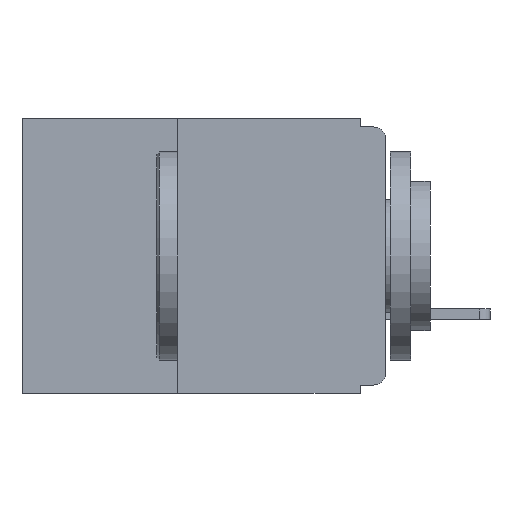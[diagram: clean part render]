
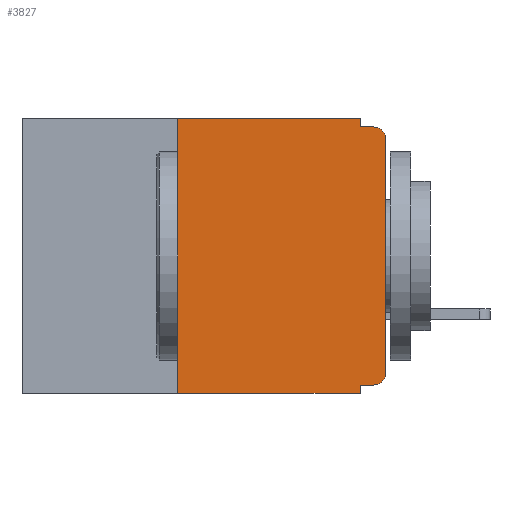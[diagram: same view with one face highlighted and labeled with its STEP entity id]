
A CAD part, left-side view. The second image highlights one B-rep face of the part: STEP entity #3827.
In plain terms, the highlighted planar face has unit normal (-1, 0, 0).
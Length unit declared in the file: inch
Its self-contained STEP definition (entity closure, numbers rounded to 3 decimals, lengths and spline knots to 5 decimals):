
#348 = AXIS2_PLACEMENT_3D ( 'NONE', #14447, #14427, #15139 ) ;
#410 = VECTOR ( 'NONE', #9246, 39.37008 ) ;
#411 = EDGE_CURVE ( 'NONE', #6225, #6337, #15366, .T. ) ;
#481 = ORIENTED_EDGE ( 'NONE', *, *, #848, .F. ) ;
#543 = EDGE_CURVE ( 'NONE', #963, #13553, #2872, .T. ) ;
#816 = CARTESIAN_POINT ( 'NONE',  ( 0., 0.437, 0. ) ) ;
#827 = LINE ( 'NONE', #11089, #410 ) ;
#848 = EDGE_CURVE ( 'NONE', #14130, #13197, #3654, .T. ) ;
#916 = VERTEX_POINT ( 'NONE', #8797 ) ;
#923 = EDGE_CURVE ( 'NONE', #6337, #13553, #6423, .T. ) ;
#963 = VERTEX_POINT ( 'NONE', #6775 ) ;
#1004 = EDGE_CURVE ( 'NONE', #14130, #6225, #8576, .T. ) ;
#1353 = CARTESIAN_POINT ( 'NONE',  ( 0., 0.031, 0. ) ) ;
#1358 = AXIS2_PLACEMENT_3D ( 'NONE', #3592, #9985, #3199 ) ;
#2254 = VECTOR ( 'NONE', #15752, 39.37008 ) ;
#2474 = VECTOR ( 'NONE', #9065, 39.37008 ) ;
#2872 = LINE ( 'NONE', #10908, #2474 ) ;
#2999 = ORIENTED_EDGE ( 'NONE', *, *, #923, .T. ) ;
#3199 = DIRECTION ( 'NONE',  ( 0., 0., -1. ) ) ;
#3592 = CARTESIAN_POINT ( 'NONE',  ( 0., 0.015, -0.025 ) ) ;
#3654 = LINE ( 'NONE', #4986, #13176 ) ;
#3827 = ADVANCED_FACE ( 'NONE', ( #10230 ), #13793, .F. ) ;
#4986 = CARTESIAN_POINT ( 'NONE',  ( 0., 0., -0.32 ) ) ;
#5029 = CARTESIAN_POINT ( 'NONE',  ( 0., 0., 0. ) ) ;
#5352 = ORIENTED_EDGE ( 'NONE', *, *, #5607, .F. ) ;
#5473 = LINE ( 'NONE', #12480, #11760 ) ;
#5557 = EDGE_CURVE ( 'NONE', #13282, #963, #5473, .T. ) ;
#5607 = EDGE_CURVE ( 'NONE', #916, #11730, #8041, .T. ) ;
#5628 = EDGE_CURVE ( 'NONE', #916, #6317, #827, .T. ) ;
#5681 = EDGE_CURVE ( 'NONE', #13197, #6317, #15749, .T. ) ;
#5975 = EDGE_LOOP ( 'NONE', ( #8987, #2999, #11660, #7120, #13309, #5352, #10160, #14050, #481, #10269 ) ) ;
#6225 = VERTEX_POINT ( 'NONE', #10763 ) ;
#6317 = VERTEX_POINT ( 'NONE', #9781 ) ;
#6337 = VERTEX_POINT ( 'NONE', #6688 ) ;
#6423 = CIRCLE ( 'NONE', #1358, 0.015 ) ;
#6459 = VECTOR ( 'NONE', #11538, 39.37008 ) ;
#6688 = CARTESIAN_POINT ( 'NONE',  ( 0., 0., -0.025 ) ) ;
#6775 = CARTESIAN_POINT ( 'NONE',  ( 0., 0.031, -0.01 ) ) ;
#7120 = ORIENTED_EDGE ( 'NONE', *, *, #5557, .F. ) ;
#7586 = DIRECTION ( 'NONE',  ( 0., 0., 1. ) ) ;
#7600 = CARTESIAN_POINT ( 'NONE',  ( 0., 0.031, -0.32 ) ) ;
#8041 = LINE ( 'NONE', #8678, #13791 ) ;
#8576 = CIRCLE ( 'NONE', #348, 0.015 ) ;
#8678 = CARTESIAN_POINT ( 'NONE',  ( 0., 0.25, -0.33 ) ) ;
#8797 = CARTESIAN_POINT ( 'NONE',  ( 0., 0.25, -0.33 ) ) ;
#8987 = ORIENTED_EDGE ( 'NONE', *, *, #411, .T. ) ;
#9065 = DIRECTION ( 'NONE',  ( 0., -1., 0. ) ) ;
#9246 = DIRECTION ( 'NONE',  ( 0., -1., 0. ) ) ;
#9781 = CARTESIAN_POINT ( 'NONE',  ( 0., 0.031, -0.33 ) ) ;
#9985 = DIRECTION ( 'NONE',  ( -1., 0., 0. ) ) ;
#10095 = CARTESIAN_POINT ( 'NONE',  ( 0., 0.015, -0.32 ) ) ;
#10146 = EDGE_CURVE ( 'NONE', #11730, #13282, #13825, .T. ) ;
#10160 = ORIENTED_EDGE ( 'NONE', *, *, #5628, .T. ) ;
#10230 = FACE_OUTER_BOUND ( 'NONE', #5975, .T. ) ;
#10269 = ORIENTED_EDGE ( 'NONE', *, *, #1004, .T. ) ;
#10763 = CARTESIAN_POINT ( 'NONE',  ( 0., 0., -0.305 ) ) ;
#10908 = CARTESIAN_POINT ( 'NONE',  ( 0., 0., -0.01 ) ) ;
#11089 = CARTESIAN_POINT ( 'NONE',  ( 0., 0.437, -0.33 ) ) ;
#11538 = DIRECTION ( 'NONE',  ( 0., 0., -1. ) ) ;
#11570 = CARTESIAN_POINT ( 'NONE',  ( 0., 0.031, -0.33 ) ) ;
#11619 = AXIS2_PLACEMENT_3D ( 'NONE', #13689, #13524, #13504 ) ;
#11660 = ORIENTED_EDGE ( 'NONE', *, *, #543, .F. ) ;
#11730 = VERTEX_POINT ( 'NONE', #12590 ) ;
#11760 = VECTOR ( 'NONE', #13904, 39.37008 ) ;
#12369 = DIRECTION ( 'NONE',  ( 0., 1., 0. ) ) ;
#12480 = CARTESIAN_POINT ( 'NONE',  ( 0., 0.031, 0. ) ) ;
#12590 = CARTESIAN_POINT ( 'NONE',  ( 0., 0.25, 0. ) ) ;
#13176 = VECTOR ( 'NONE', #12369, 39.37008 ) ;
#13197 = VERTEX_POINT ( 'NONE', #7600 ) ;
#13282 = VERTEX_POINT ( 'NONE', #1353 ) ;
#13309 = ORIENTED_EDGE ( 'NONE', *, *, #10146, .F. ) ;
#13447 = VECTOR ( 'NONE', #15666, 39.37008 ) ;
#13504 = DIRECTION ( 'NONE',  ( 0., 0., -1. ) ) ;
#13524 = DIRECTION ( 'NONE',  ( 1., 0., 0. ) ) ;
#13553 = VERTEX_POINT ( 'NONE', #14984 ) ;
#13689 = CARTESIAN_POINT ( 'NONE',  ( 0., 0.437, 0. ) ) ;
#13791 = VECTOR ( 'NONE', #7586, 39.37008 ) ;
#13793 = PLANE ( 'NONE',  #11619 ) ;
#13825 = LINE ( 'NONE', #816, #13447 ) ;
#13904 = DIRECTION ( 'NONE',  ( 0., 0., -1. ) ) ;
#14050 = ORIENTED_EDGE ( 'NONE', *, *, #5681, .F. ) ;
#14130 = VERTEX_POINT ( 'NONE', #10095 ) ;
#14427 = DIRECTION ( 'NONE',  ( -1., 0., 0. ) ) ;
#14447 = CARTESIAN_POINT ( 'NONE',  ( 0., 0.015, -0.305 ) ) ;
#14984 = CARTESIAN_POINT ( 'NONE',  ( 0., 0.015, -0.01 ) ) ;
#15139 = DIRECTION ( 'NONE',  ( 0., 0., -1. ) ) ;
#15366 = LINE ( 'NONE', #5029, #2254 ) ;
#15666 = DIRECTION ( 'NONE',  ( 0., -1., 0. ) ) ;
#15749 = LINE ( 'NONE', #11570, #6459 ) ;
#15752 = DIRECTION ( 'NONE',  ( 0., 0., 1. ) ) ;
